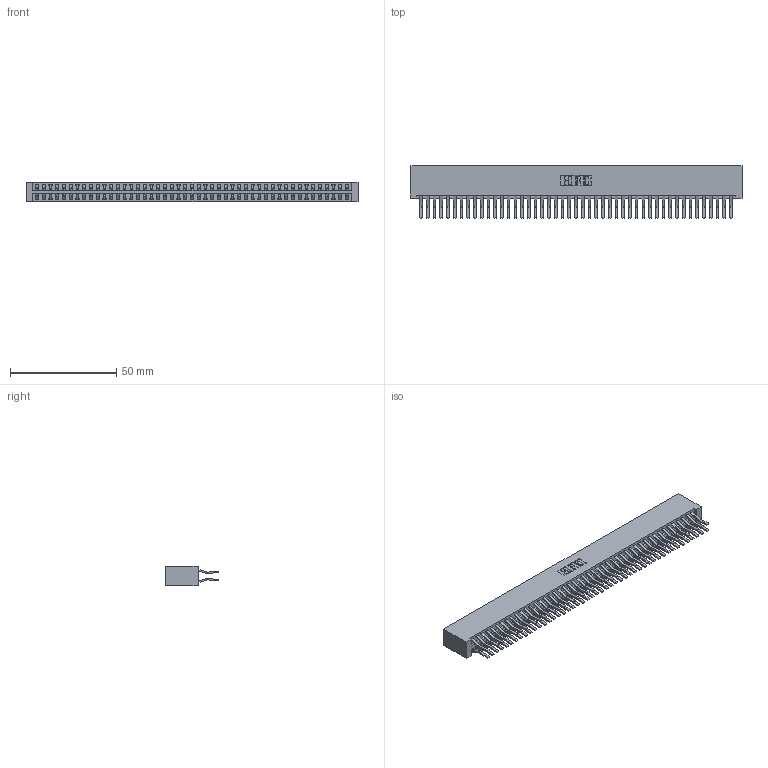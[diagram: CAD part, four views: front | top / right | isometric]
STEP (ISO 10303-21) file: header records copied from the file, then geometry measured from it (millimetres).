
FILE_DESCRIPTION (( 'STEP AP203' ), '1' );
FILE_NAME ('346-094-560-201.STEP', '2022-05-26T15:25:34', ( '' ), ( '' ), 'SwSTEP 2.0', 'SolidWorks 2020', '' );
FILE_SCHEMA (( 'CONFIG_CONTROL_DESIGN' ));
Length unit declared in the file: inch
Products named in the file (3): 346-094-560-201; 345-292-001_560 Tail; 346 Part_No Mounting Lugs
Assembly tree (95 placements, depth 2):
  346-094-560-201
    346 Part_No Mounting Lugs
    345-292-001_560 Tail  x94
Bounding box: 156.46 x 24.78 x 9.4 mm (x, y, z)
Volume: 16485.4 mm3; surface area: 24545.9 mm2
Topology: 95 solids, 95 shells, 5190 faces, 15439 edges, 10166 vertices
Faces by surface type: plane 3362, cylinder 1828
Entity records: 29811 total; most frequent: CARTESIAN_POINT 4904, ORIENTED_EDGE 4838, DIRECTION 4371, EDGE_CURVE 2419, VECTOR 2103, LINE 2103, VERTEX_POINT 1610, AXIS2_PLACEMENT_3D 1134
